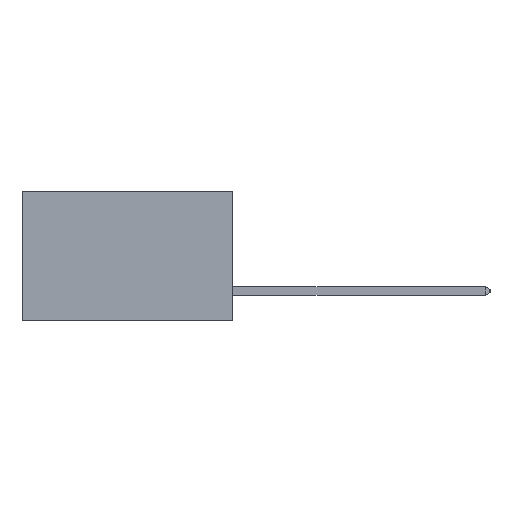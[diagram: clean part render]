
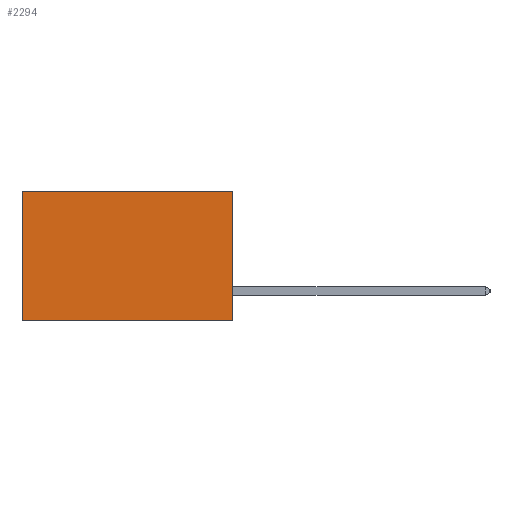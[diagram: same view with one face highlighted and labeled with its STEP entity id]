
A CAD part, left-side view. The second image highlights one B-rep face of the part: STEP entity #2294.
In plain terms, the highlighted planar face has unit normal (-1, 0, 0).
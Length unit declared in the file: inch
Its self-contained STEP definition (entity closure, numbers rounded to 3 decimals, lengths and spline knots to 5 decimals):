
#214 = EDGE_CURVE ( 'NONE', #7003, #11911, #4539, .T. ) ;
#344 = VECTOR ( 'NONE', #9803, 39.37008 ) ;
#1407 = LINE ( 'NONE', #12512, #5511 ) ;
#2294 = ADVANCED_FACE ( 'NONE', ( #12451 ), #2924, .F. ) ;
#2924 = PLANE ( 'NONE',  #8166 ) ;
#3082 = VERTEX_POINT ( 'NONE', #5589 ) ;
#4415 = LINE ( 'NONE', #11576, #344 ) ;
#4539 = LINE ( 'NONE', #18138, #7519 ) ;
#4978 = EDGE_CURVE ( 'NONE', #14649, #11911, #8387, .T. ) ;
#5056 = DIRECTION ( 'NONE',  ( 1., 0., 0. ) ) ;
#5511 = VECTOR ( 'NONE', #17597, 39.37008 ) ;
#5589 = CARTESIAN_POINT ( 'NONE',  ( 0.2875, 0., 0. ) ) ;
#6126 = ORIENTED_EDGE ( 'NONE', *, *, #8234, .F. ) ;
#7003 = VERTEX_POINT ( 'NONE', #21754 ) ;
#7389 = EDGE_LOOP ( 'NONE', ( #20822, #13964, #6126, #7663 ) ) ;
#7519 = VECTOR ( 'NONE', #18909, 39.37008 ) ;
#7663 = ORIENTED_EDGE ( 'NONE', *, *, #8643, .T. ) ;
#7827 = VECTOR ( 'NONE', #16392, 39.37008 ) ;
#8166 = AXIS2_PLACEMENT_3D ( 'NONE', #18299, #5056, #21673 ) ;
#8234 = EDGE_CURVE ( 'NONE', #3082, #14649, #4415, .T. ) ;
#8387 = LINE ( 'NONE', #18591, #7827 ) ;
#8643 = EDGE_CURVE ( 'NONE', #3082, #7003, #1407, .T. ) ;
#8879 = CARTESIAN_POINT ( 'NONE',  ( 0.2875, 0., -0.37 ) ) ;
#9803 = DIRECTION ( 'NONE',  ( 0., 0., -1. ) ) ;
#11576 = CARTESIAN_POINT ( 'NONE',  ( 0.2875, 0., 0. ) ) ;
#11911 = VERTEX_POINT ( 'NONE', #16842 ) ;
#12451 = FACE_OUTER_BOUND ( 'NONE', #7389, .T. ) ;
#12512 = CARTESIAN_POINT ( 'NONE',  ( 0.2875, 0., 0. ) ) ;
#13964 = ORIENTED_EDGE ( 'NONE', *, *, #4978, .F. ) ;
#14649 = VERTEX_POINT ( 'NONE', #8879 ) ;
#16392 = DIRECTION ( 'NONE',  ( 0., 1., 0. ) ) ;
#16842 = CARTESIAN_POINT ( 'NONE',  ( 0.2875, 0.6, -0.37 ) ) ;
#17597 = DIRECTION ( 'NONE',  ( 0., 1., 0. ) ) ;
#18138 = CARTESIAN_POINT ( 'NONE',  ( 0.2875, 0.6, 0. ) ) ;
#18299 = CARTESIAN_POINT ( 'NONE',  ( 0.2875, 0., 0. ) ) ;
#18591 = CARTESIAN_POINT ( 'NONE',  ( 0.2875, 0., -0.37 ) ) ;
#18909 = DIRECTION ( 'NONE',  ( 0., 0., -1. ) ) ;
#20822 = ORIENTED_EDGE ( 'NONE', *, *, #214, .T. ) ;
#21673 = DIRECTION ( 'NONE',  ( 0., 0., -1. ) ) ;
#21754 = CARTESIAN_POINT ( 'NONE',  ( 0.2875, 0.6, 0. ) ) ;
